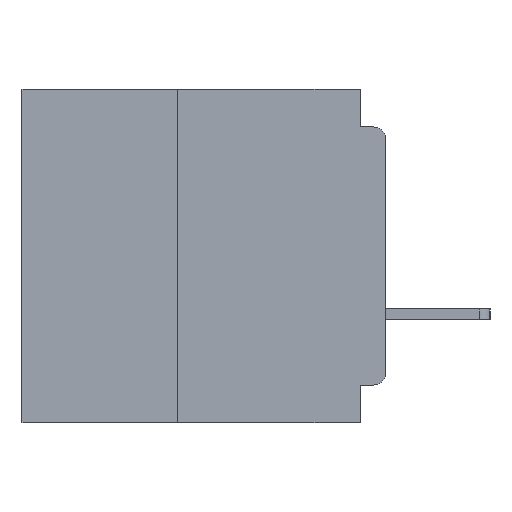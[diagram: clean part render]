
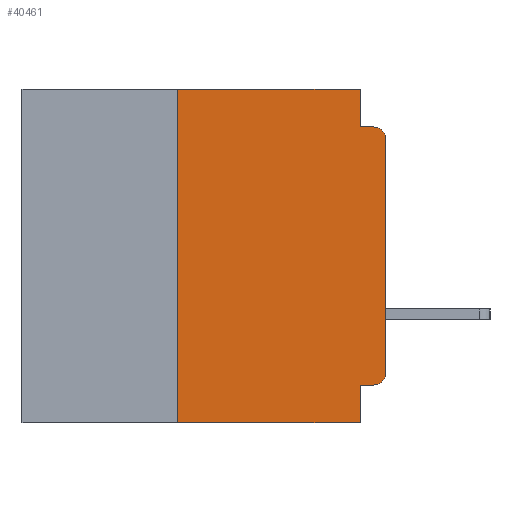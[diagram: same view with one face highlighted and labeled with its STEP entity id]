
A CAD part, left-side view. The second image highlights one B-rep face of the part: STEP entity #40461.
In plain terms, the highlighted planar face has unit normal (-1, 0, 0).
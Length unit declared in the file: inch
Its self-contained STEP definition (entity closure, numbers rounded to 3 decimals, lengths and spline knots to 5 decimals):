
#1939 = VERTEX_POINT ( 'NONE', #26468 ) ;
#3043 = AXIS2_PLACEMENT_3D ( 'NONE', #22201, #52523, #26563 ) ;
#4271 = CARTESIAN_POINT ( 'NONE',  ( 0., 0.031, -0.355 ) ) ;
#5693 = CARTESIAN_POINT ( 'NONE',  ( 0., 0.031, 0. ) ) ;
#5873 = LINE ( 'NONE', #36111, #27544 ) ;
#5967 = EDGE_CURVE ( 'NONE', #31510, #19263, #7929, .T. ) ;
#6026 = EDGE_CURVE ( 'NONE', #10117, #18154, #49951, .T. ) ;
#7543 = LINE ( 'NONE', #21672, #39499 ) ;
#7929 = LINE ( 'NONE', #28598, #16703 ) ;
#8100 = EDGE_LOOP ( 'NONE', ( #49637, #35810, #52563, #12615, #11306, #11631, #40226, #46796, #32661, #42220 ) ) ;
#9149 = PLANE ( 'NONE',  #3043 ) ;
#10042 = EDGE_CURVE ( 'NONE', #13134, #32789, #17798, .T. ) ;
#10117 = VERTEX_POINT ( 'NONE', #48907 ) ;
#10555 = FACE_OUTER_BOUND ( 'NONE', #8100, .T. ) ;
#11306 = ORIENTED_EDGE ( 'NONE', *, *, #19742, .F. ) ;
#11587 = VERTEX_POINT ( 'NONE', #5693 ) ;
#11631 = ORIENTED_EDGE ( 'NONE', *, *, #10042, .F. ) ;
#11937 = CARTESIAN_POINT ( 'NONE',  ( 0., 0.015, -0.34 ) ) ;
#12615 = ORIENTED_EDGE ( 'NONE', *, *, #44821, .F. ) ;
#13134 = VERTEX_POINT ( 'NONE', #16281 ) ;
#13898 = VERTEX_POINT ( 'NONE', #55306 ) ;
#16199 = VERTEX_POINT ( 'NONE', #19478 ) ;
#16281 = CARTESIAN_POINT ( 'NONE',  ( 0., 0.25, -0.4 ) ) ;
#16292 = DIRECTION ( 'NONE',  ( 0., 0., -1. ) ) ;
#16703 = VECTOR ( 'NONE', #41788, 39.37008 ) ;
#17208 = DIRECTION ( 'NONE',  ( 0., 0., 1. ) ) ;
#17798 = LINE ( 'NONE', #30121, #51003 ) ;
#18132 = DIRECTION ( 'NONE',  ( 0., -1., 0. ) ) ;
#18154 = VERTEX_POINT ( 'NONE', #35763 ) ;
#19263 = VERTEX_POINT ( 'NONE', #53544 ) ;
#19478 = CARTESIAN_POINT ( 'NONE',  ( 0., 0., -0.06 ) ) ;
#19742 = EDGE_CURVE ( 'NONE', #32789, #11587, #38462, .T. ) ;
#21352 = CIRCLE ( 'NONE', #26732, 0.015 ) ;
#21672 = CARTESIAN_POINT ( 'NONE',  ( 0., 0., -0.355 ) ) ;
#22201 = CARTESIAN_POINT ( 'NONE',  ( 0., 0.437, 0. ) ) ;
#22850 = LINE ( 'NONE', #25349, #25561 ) ;
#23020 = CARTESIAN_POINT ( 'NONE',  ( 0., 0.437, 0. ) ) ;
#23952 = DIRECTION ( 'NONE',  ( -1., 0., 0. ) ) ;
#25349 = CARTESIAN_POINT ( 'NONE',  ( 0., 0.031, 0. ) ) ;
#25561 = VECTOR ( 'NONE', #55652, 39.37008 ) ;
#26468 = CARTESIAN_POINT ( 'NONE',  ( 0., 0.015, -0.355 ) ) ;
#26563 = DIRECTION ( 'NONE',  ( 0., 0., -1. ) ) ;
#26732 = AXIS2_PLACEMENT_3D ( 'NONE', #49943, #23952, #54244 ) ;
#26829 = VECTOR ( 'NONE', #31816, 39.37008 ) ;
#27544 = VECTOR ( 'NONE', #40455, 39.37008 ) ;
#28598 = CARTESIAN_POINT ( 'NONE',  ( 0., 0.031, -0.4 ) ) ;
#30121 = CARTESIAN_POINT ( 'NONE',  ( 0., 0.25, -0.4 ) ) ;
#30489 = CARTESIAN_POINT ( 'NONE',  ( 0., 0.25, 0. ) ) ;
#31510 = VERTEX_POINT ( 'NONE', #4271 ) ;
#31816 = DIRECTION ( 'NONE',  ( 0., -1., 0. ) ) ;
#32661 = ORIENTED_EDGE ( 'NONE', *, *, #34316, .F. ) ;
#32789 = VERTEX_POINT ( 'NONE', #30489 ) ;
#34316 = EDGE_CURVE ( 'NONE', #1939, #31510, #7543, .T. ) ;
#34772 = EDGE_CURVE ( 'NONE', #1939, #13898, #50853, .T. ) ;
#35665 = EDGE_CURVE ( 'NONE', #13134, #19263, #48070, .T. ) ;
#35763 = CARTESIAN_POINT ( 'NONE',  ( 0., 0.015, -0.045 ) ) ;
#35810 = ORIENTED_EDGE ( 'NONE', *, *, #52522, .T. ) ;
#36111 = CARTESIAN_POINT ( 'NONE',  ( 0., 0., 0. ) ) ;
#38462 = LINE ( 'NONE', #23020, #26829 ) ;
#39499 = VECTOR ( 'NONE', #43374, 39.37008 ) ;
#39832 = CARTESIAN_POINT ( 'NONE',  ( 0., 0.437, -0.4 ) ) ;
#40226 = ORIENTED_EDGE ( 'NONE', *, *, #35665, .T. ) ;
#40455 = DIRECTION ( 'NONE',  ( 0., 0., 1. ) ) ;
#40461 = ADVANCED_FACE ( 'NONE', ( #10555 ), #9149, .F. ) ;
#41788 = DIRECTION ( 'NONE',  ( 0., 0., -1. ) ) ;
#42220 = ORIENTED_EDGE ( 'NONE', *, *, #34772, .T. ) ;
#42374 = DIRECTION ( 'NONE',  ( -1., 0., 0. ) ) ;
#43374 = DIRECTION ( 'NONE',  ( 0., 1., 0. ) ) ;
#44821 = EDGE_CURVE ( 'NONE', #11587, #10117, #22850, .T. ) ;
#46288 = DIRECTION ( 'NONE',  ( 0., -1., 0. ) ) ;
#46722 = VECTOR ( 'NONE', #18132, 39.37008 ) ;
#46796 = ORIENTED_EDGE ( 'NONE', *, *, #5967, .F. ) ;
#48070 = LINE ( 'NONE', #39832, #46722 ) ;
#48245 = AXIS2_PLACEMENT_3D ( 'NONE', #11937, #42374, #16292 ) ;
#48619 = VECTOR ( 'NONE', #46288, 39.37008 ) ;
#48907 = CARTESIAN_POINT ( 'NONE',  ( 0., 0.031, -0.045 ) ) ;
#49637 = ORIENTED_EDGE ( 'NONE', *, *, #51770, .T. ) ;
#49943 = CARTESIAN_POINT ( 'NONE',  ( 0., 0.015, -0.06 ) ) ;
#49951 = LINE ( 'NONE', #50581, #48619 ) ;
#50581 = CARTESIAN_POINT ( 'NONE',  ( 0., 0., -0.045 ) ) ;
#50853 = CIRCLE ( 'NONE', #48245, 0.015 ) ;
#51003 = VECTOR ( 'NONE', #17208, 39.37008 ) ;
#51770 = EDGE_CURVE ( 'NONE', #13898, #16199, #5873, .T. ) ;
#52522 = EDGE_CURVE ( 'NONE', #16199, #18154, #21352, .T. ) ;
#52523 = DIRECTION ( 'NONE',  ( 1., 0., 0. ) ) ;
#52563 = ORIENTED_EDGE ( 'NONE', *, *, #6026, .F. ) ;
#53544 = CARTESIAN_POINT ( 'NONE',  ( 0., 0.031, -0.4 ) ) ;
#54244 = DIRECTION ( 'NONE',  ( 0., 0., -1. ) ) ;
#55306 = CARTESIAN_POINT ( 'NONE',  ( 0., 0., -0.34 ) ) ;
#55652 = DIRECTION ( 'NONE',  ( 0., 0., -1. ) ) ;
